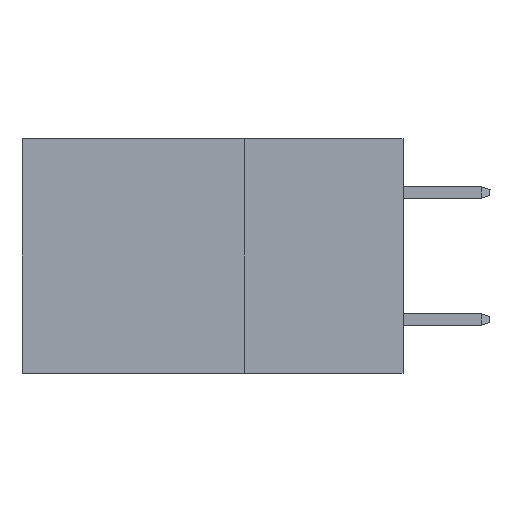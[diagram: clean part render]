
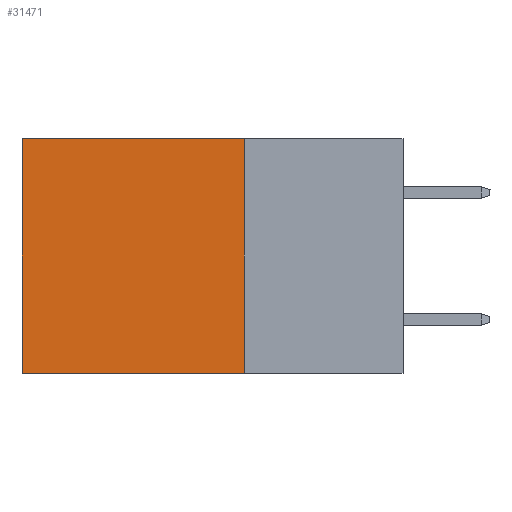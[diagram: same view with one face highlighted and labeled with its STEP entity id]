
A CAD part, left-side view. The second image highlights one B-rep face of the part: STEP entity #31471.
In plain terms, the highlighted planar face has unit normal (-1, 0, 0).
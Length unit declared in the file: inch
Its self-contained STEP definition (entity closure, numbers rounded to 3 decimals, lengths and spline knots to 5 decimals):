
#220 = AXIS2_PLACEMENT_3D ( 'NONE', #19717, #13848, #4713 ) ;
#1462 = FACE_OUTER_BOUND ( 'NONE', #19001, .T. ) ;
#2142 = CARTESIAN_POINT ( 'NONE',  ( 0.2875, 0.25, 0. ) ) ;
#4713 = DIRECTION ( 'NONE',  ( 0., 0., -1. ) ) ;
#5275 = ORIENTED_EDGE ( 'NONE', *, *, #14018, .T. ) ;
#5613 = CARTESIAN_POINT ( 'NONE',  ( 0.2875, 0.6, -0.37 ) ) ;
#5684 = EDGE_CURVE ( 'NONE', #32993, #6992, #35029, .T. ) ;
#6701 = CARTESIAN_POINT ( 'NONE',  ( 0.2875, 0.25, -0.37 ) ) ;
#6992 = VERTEX_POINT ( 'NONE', #5613 ) ;
#7007 = DIRECTION ( 'NONE',  ( 0., 0., -1. ) ) ;
#9580 = EDGE_CURVE ( 'NONE', #29905, #39984, #11936, .T. ) ;
#11936 = LINE ( 'NONE', #37285, #26535 ) ;
#12580 = CARTESIAN_POINT ( 'NONE',  ( 0.2875, 0.25, 0. ) ) ;
#13848 = DIRECTION ( 'NONE',  ( 1., 0., 0. ) ) ;
#14018 = EDGE_CURVE ( 'NONE', #29905, #32993, #39898, .T. ) ;
#14094 = CARTESIAN_POINT ( 'NONE',  ( 0.2875, 0.25, -0.37 ) ) ;
#15737 = CARTESIAN_POINT ( 'NONE',  ( 0.2875, 0.6, 0. ) ) ;
#16028 = CARTESIAN_POINT ( 'NONE',  ( 0.2875, 0.6, 0. ) ) ;
#17253 = VECTOR ( 'NONE', #7007, 39.37008 ) ;
#17608 = ORIENTED_EDGE ( 'NONE', *, *, #9580, .F. ) ;
#18818 = VECTOR ( 'NONE', #31455, 39.37008 ) ;
#19001 = EDGE_LOOP ( 'NONE', ( #29556, #26143, #17608, #5275 ) ) ;
#19193 = DIRECTION ( 'NONE',  ( 0., 0., -1. ) ) ;
#19717 = CARTESIAN_POINT ( 'NONE',  ( 0.2875, 0.25, 0. ) ) ;
#21533 = LINE ( 'NONE', #6701, #18818 ) ;
#23442 = VECTOR ( 'NONE', #24256, 39.37008 ) ;
#24256 = DIRECTION ( 'NONE',  ( 0., 1., 0. ) ) ;
#26143 = ORIENTED_EDGE ( 'NONE', *, *, #27177, .F. ) ;
#26535 = VECTOR ( 'NONE', #19193, 39.37008 ) ;
#27177 = EDGE_CURVE ( 'NONE', #39984, #6992, #21533, .T. ) ;
#29556 = ORIENTED_EDGE ( 'NONE', *, *, #5684, .T. ) ;
#29905 = VERTEX_POINT ( 'NONE', #12580 ) ;
#31455 = DIRECTION ( 'NONE',  ( 0., 1., 0. ) ) ;
#31471 = ADVANCED_FACE ( 'NONE', ( #1462 ), #34978, .F. ) ;
#32993 = VERTEX_POINT ( 'NONE', #16028 ) ;
#34978 = PLANE ( 'NONE',  #220 ) ;
#35029 = LINE ( 'NONE', #15737, #17253 ) ;
#37285 = CARTESIAN_POINT ( 'NONE',  ( 0.2875, 0.25, 0. ) ) ;
#39898 = LINE ( 'NONE', #2142, #23442 ) ;
#39984 = VERTEX_POINT ( 'NONE', #14094 ) ;
